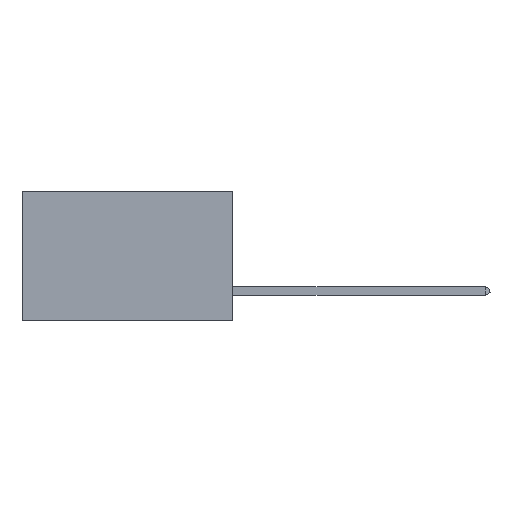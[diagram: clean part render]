
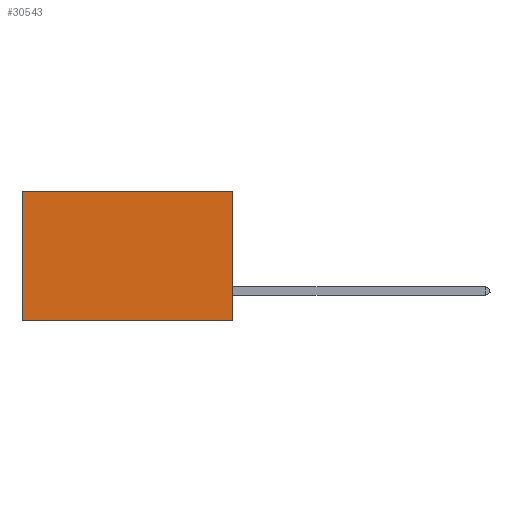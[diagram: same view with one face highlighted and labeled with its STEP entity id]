
A CAD part, left-side view. The second image highlights one B-rep face of the part: STEP entity #30543.
In plain terms, the highlighted planar face has unit normal (-1, 0, 0).
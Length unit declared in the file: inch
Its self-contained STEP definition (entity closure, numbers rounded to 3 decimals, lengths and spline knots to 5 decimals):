
#2861 = PLANE ( 'NONE',  #30810 ) ;
#3330 = VECTOR ( 'NONE', #21310, 39.37008 ) ;
#3727 = CARTESIAN_POINT ( 'NONE',  ( 0.2875, 0., 0. ) ) ;
#3855 = LINE ( 'NONE', #42480, #38500 ) ;
#4342 = VERTEX_POINT ( 'NONE', #42344 ) ;
#6754 = DIRECTION ( 'NONE',  ( 1., 0., 0. ) ) ;
#7292 = DIRECTION ( 'NONE',  ( 0., 0., -1. ) ) ;
#10910 = VERTEX_POINT ( 'NONE', #19289 ) ;
#14640 = CARTESIAN_POINT ( 'NONE',  ( 0.2875, 0., 0. ) ) ;
#14954 = LINE ( 'NONE', #3727, #3330 ) ;
#15482 = DIRECTION ( 'NONE',  ( 0., 1., 0. ) ) ;
#17464 = CARTESIAN_POINT ( 'NONE',  ( 0.2875, 0., -0.37 ) ) ;
#17537 = ORIENTED_EDGE ( 'NONE', *, *, #23011, .T. ) ;
#18255 = ORIENTED_EDGE ( 'NONE', *, *, #22989, .T. ) ;
#19289 = CARTESIAN_POINT ( 'NONE',  ( 0.2875, 0.6, 0. ) ) ;
#21310 = DIRECTION ( 'NONE',  ( 0., 1., 0. ) ) ;
#22220 = EDGE_CURVE ( 'NONE', #4342, #38271, #41358, .T. ) ;
#22989 = EDGE_CURVE ( 'NONE', #4342, #10910, #14954, .T. ) ;
#23011 = EDGE_CURVE ( 'NONE', #10910, #30024, #3855, .T. ) ;
#23972 = CARTESIAN_POINT ( 'NONE',  ( 0.2875, 0., 0. ) ) ;
#24467 = CARTESIAN_POINT ( 'NONE',  ( 0.2875, 0.6, -0.37 ) ) ;
#25705 = CARTESIAN_POINT ( 'NONE',  ( 0.2875, 0., -0.37 ) ) ;
#27312 = VECTOR ( 'NONE', #15482, 39.37008 ) ;
#28909 = LINE ( 'NONE', #25705, #27312 ) ;
#29336 = EDGE_LOOP ( 'NONE', ( #17537, #32290, #36868, #18255 ) ) ;
#29760 = VECTOR ( 'NONE', #30832, 39.37008 ) ;
#30024 = VERTEX_POINT ( 'NONE', #24467 ) ;
#30543 = ADVANCED_FACE ( 'NONE', ( #42281 ), #2861, .F. ) ;
#30810 = AXIS2_PLACEMENT_3D ( 'NONE', #14640, #6754, #34835 ) ;
#30832 = DIRECTION ( 'NONE',  ( 0., 0., -1. ) ) ;
#32290 = ORIENTED_EDGE ( 'NONE', *, *, #34764, .F. ) ;
#34764 = EDGE_CURVE ( 'NONE', #38271, #30024, #28909, .T. ) ;
#34835 = DIRECTION ( 'NONE',  ( 0., 0., -1. ) ) ;
#36868 = ORIENTED_EDGE ( 'NONE', *, *, #22220, .F. ) ;
#38271 = VERTEX_POINT ( 'NONE', #17464 ) ;
#38500 = VECTOR ( 'NONE', #7292, 39.37008 ) ;
#41358 = LINE ( 'NONE', #23972, #29760 ) ;
#42281 = FACE_OUTER_BOUND ( 'NONE', #29336, .T. ) ;
#42344 = CARTESIAN_POINT ( 'NONE',  ( 0.2875, 0., 0. ) ) ;
#42480 = CARTESIAN_POINT ( 'NONE',  ( 0.2875, 0.6, 0. ) ) ;
